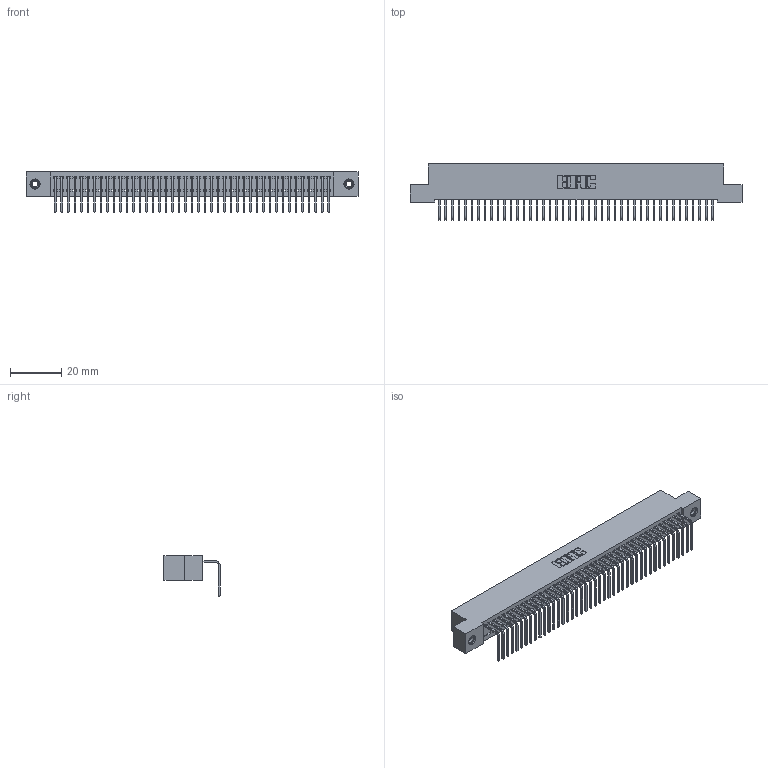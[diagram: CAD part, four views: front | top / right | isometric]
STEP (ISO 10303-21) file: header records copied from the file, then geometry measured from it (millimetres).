
FILE_DESCRIPTION (( 'STEP AP203' ), '1' );
FILE_NAME ('342-043-558-108.STEP', '2018-08-12T14:03:03', ( '' ), ( '' ), 'SwSTEP 2.0', 'SolidWorks 2016', '' );
FILE_SCHEMA (( 'CONFIG_CONTROL_DESIGN' ));
Length unit declared in the file: inch
Products named in the file (4): 342-043-558-108; 342 Part_TI; 345-292-001_558 Tail - 2; 345-250-001_345-250-003-102
Assembly tree (46 placements, depth 2):
  342-043-558-108
    342 Part_TI
    345-292-001_558 Tail - 2  x43
    345-250-001_345-250-003-102  x2
Bounding box: 129.54 x 21.91 x 15.62 mm (x, y, z)
Volume: 11499.3 mm3; surface area: 17736.4 mm2
Topology: 46 solids, 46 shells, 2750 faces, 8261 edges, 5442 vertices
Faces by surface type: plane 1990, cylinder 744, cone 12, torus 4
Entity records: 27296 total; most frequent: CARTESIAN_POINT 4690, ORIENTED_EDGE 4662, DIRECTION 3987, EDGE_CURVE 2331, VECTOR 2183, LINE 2183, VERTEX_POINT 1548, AXIS2_PLACEMENT_3D 902
